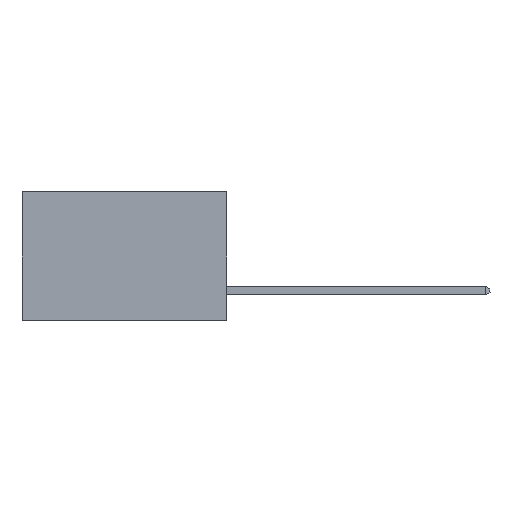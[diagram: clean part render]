
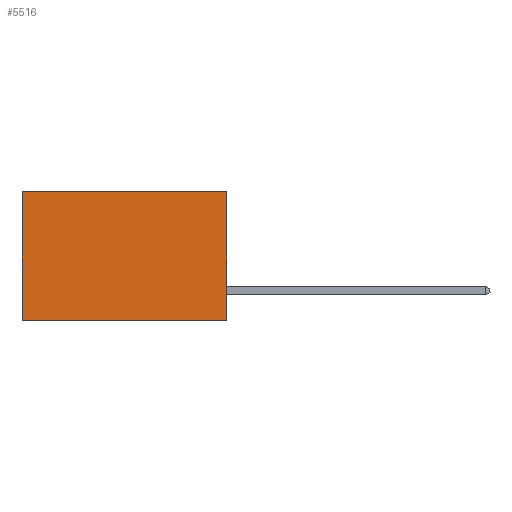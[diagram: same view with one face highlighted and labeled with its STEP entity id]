
A CAD part, left-side view. The second image highlights one B-rep face of the part: STEP entity #5516.
In plain terms, the highlighted planar face has unit normal (-1, 0, 0).
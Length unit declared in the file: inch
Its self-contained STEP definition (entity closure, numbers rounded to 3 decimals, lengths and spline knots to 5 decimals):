
#558 = EDGE_LOOP ( 'NONE', ( #883, #2084, #1877, #8204 ) ) ;
#832 = CARTESIAN_POINT ( 'NONE',  ( 0.277, 0., 0. ) ) ;
#883 = ORIENTED_EDGE ( 'NONE', *, *, #1924, .T. ) ;
#1384 = EDGE_CURVE ( 'NONE', #1524, #5593, #2032, .T. ) ;
#1524 = VERTEX_POINT ( 'NONE', #1911 ) ;
#1594 = DIRECTION ( 'NONE',  ( 0., 1., 0. ) ) ;
#1877 = ORIENTED_EDGE ( 'NONE', *, *, #4783, .F. ) ;
#1911 = CARTESIAN_POINT ( 'NONE',  ( 0.277, 0., -0.37 ) ) ;
#1924 = EDGE_CURVE ( 'NONE', #7470, #5593, #9120, .T. ) ;
#2032 = LINE ( 'NONE', #6539, #7416 ) ;
#2084 = ORIENTED_EDGE ( 'NONE', *, *, #1384, .F. ) ;
#2313 = CARTESIAN_POINT ( 'NONE',  ( 0.277, 0.59, 0. ) ) ;
#2550 = CARTESIAN_POINT ( 'NONE',  ( 0.277, 0.59, -0.37 ) ) ;
#3379 = VECTOR ( 'NONE', #8643, 39.37008 ) ;
#3574 = VECTOR ( 'NONE', #1594, 39.37008 ) ;
#3632 = EDGE_CURVE ( 'NONE', #6138, #7470, #7285, .T. ) ;
#4170 = LINE ( 'NONE', #5356, #7640 ) ;
#4363 = FACE_OUTER_BOUND ( 'NONE', #558, .T. ) ;
#4430 = CARTESIAN_POINT ( 'NONE',  ( 0.277, 0., 0. ) ) ;
#4783 = EDGE_CURVE ( 'NONE', #6138, #1524, #4170, .T. ) ;
#5356 = CARTESIAN_POINT ( 'NONE',  ( 0.277, 0., -0.37 ) ) ;
#5516 = ADVANCED_FACE ( 'NONE', ( #4363 ), #8502, .F. ) ;
#5593 = VERTEX_POINT ( 'NONE', #8189 ) ;
#5803 = DIRECTION ( 'NONE',  ( 0., 0., -1. ) ) ;
#6138 = VERTEX_POINT ( 'NONE', #4430 ) ;
#6539 = CARTESIAN_POINT ( 'NONE',  ( 0.277, 0., -0.37 ) ) ;
#7285 = LINE ( 'NONE', #832, #3574 ) ;
#7416 = VECTOR ( 'NONE', #8522, 39.37008 ) ;
#7470 = VERTEX_POINT ( 'NONE', #2313 ) ;
#7640 = VECTOR ( 'NONE', #5803, 39.37008 ) ;
#7786 = AXIS2_PLACEMENT_3D ( 'NONE', #8579, #8492, #8479 ) ;
#8189 = CARTESIAN_POINT ( 'NONE',  ( 0.277, 0.59, -0.37 ) ) ;
#8204 = ORIENTED_EDGE ( 'NONE', *, *, #3632, .T. ) ;
#8479 = DIRECTION ( 'NONE',  ( 0., 0., -1. ) ) ;
#8492 = DIRECTION ( 'NONE',  ( 1., 0., 0. ) ) ;
#8502 = PLANE ( 'NONE',  #7786 ) ;
#8522 = DIRECTION ( 'NONE',  ( 0., 1., 0. ) ) ;
#8579 = CARTESIAN_POINT ( 'NONE',  ( 0.277, 0., -0.37 ) ) ;
#8643 = DIRECTION ( 'NONE',  ( 0., 0., -1. ) ) ;
#9120 = LINE ( 'NONE', #2550, #3379 ) ;
